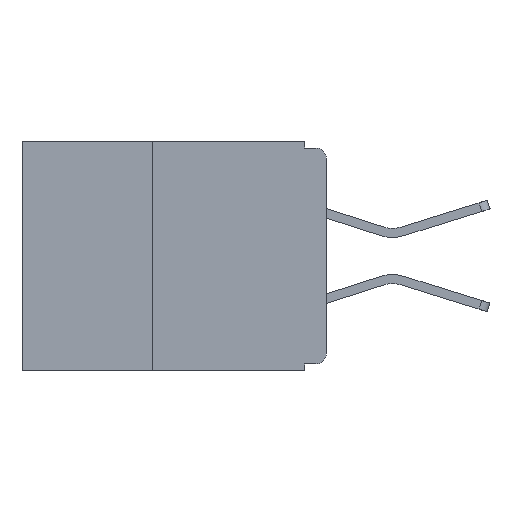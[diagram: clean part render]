
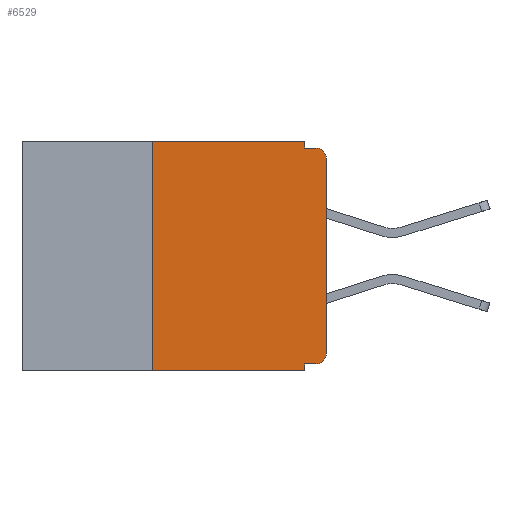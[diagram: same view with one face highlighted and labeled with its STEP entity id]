
A CAD part, left-side view. The second image highlights one B-rep face of the part: STEP entity #6529.
In plain terms, the highlighted planar face has unit normal (-1, 0, 0).
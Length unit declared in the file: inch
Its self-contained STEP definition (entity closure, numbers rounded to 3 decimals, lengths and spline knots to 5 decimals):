
#220 = ORIENTED_EDGE ( 'NONE', *, *, #1841, .T. ) ;
#854 = DIRECTION ( 'NONE',  ( 0., 0., -1. ) ) ;
#867 = CARTESIAN_POINT ( 'NONE',  ( 0., 0.25, -0.33 ) ) ;
#914 = CARTESIAN_POINT ( 'NONE',  ( 0., 0., -0.305 ) ) ;
#943 = DIRECTION ( 'NONE',  ( 0., 0., 1. ) ) ;
#957 = DIRECTION ( 'NONE',  ( -1., 0., 0. ) ) ;
#1030 = CARTESIAN_POINT ( 'NONE',  ( 0., 0.015, -0.305 ) ) ;
#1179 = LINE ( 'NONE', #15894, #25919 ) ;
#1271 = EDGE_CURVE ( 'NONE', #3011, #22748, #14163, .T. ) ;
#1357 = VECTOR ( 'NONE', #10942, 39.37008 ) ;
#1841 = EDGE_CURVE ( 'NONE', #8660, #22748, #8854, .T. ) ;
#1906 = AXIS2_PLACEMENT_3D ( 'NONE', #6302, #23555, #6839 ) ;
#1946 = ORIENTED_EDGE ( 'NONE', *, *, #25654, .T. ) ;
#2000 = CARTESIAN_POINT ( 'NONE',  ( 0., 0.031, 0. ) ) ;
#2890 = VECTOR ( 'NONE', #6925, 39.37008 ) ;
#3011 = VERTEX_POINT ( 'NONE', #15154 ) ;
#3528 = CARTESIAN_POINT ( 'NONE',  ( 0., 0.015, -0.01 ) ) ;
#3566 = EDGE_CURVE ( 'NONE', #28428, #23435, #24831, .T. ) ;
#3914 = DIRECTION ( 'NONE',  ( 0., 0., 1. ) ) ;
#4396 = FACE_OUTER_BOUND ( 'NONE', #19250, .T. ) ;
#4990 = CARTESIAN_POINT ( 'NONE',  ( 0., 0., -0.32 ) ) ;
#5442 = VECTOR ( 'NONE', #26007, 39.37008 ) ;
#5849 = AXIS2_PLACEMENT_3D ( 'NONE', #1030, #957, #854 ) ;
#5925 = ORIENTED_EDGE ( 'NONE', *, *, #29045, .F. ) ;
#6224 = CARTESIAN_POINT ( 'NONE',  ( 0., 0.25, 0. ) ) ;
#6302 = CARTESIAN_POINT ( 'NONE',  ( 0., 0.015, -0.025 ) ) ;
#6384 = EDGE_CURVE ( 'NONE', #9688, #9881, #13815, .T. ) ;
#6529 = ADVANCED_FACE ( 'NONE', ( #4396 ), #29319, .F. ) ;
#6839 = DIRECTION ( 'NONE',  ( 0., 0., -1. ) ) ;
#6925 = DIRECTION ( 'NONE',  ( 0., -1., 0. ) ) ;
#8288 = VECTOR ( 'NONE', #17057, 39.37008 ) ;
#8456 = VECTOR ( 'NONE', #25590, 39.37008 ) ;
#8660 = VERTEX_POINT ( 'NONE', #22276 ) ;
#8854 = CIRCLE ( 'NONE', #1906, 0.015 ) ;
#9190 = LINE ( 'NONE', #13715, #8456 ) ;
#9688 = VERTEX_POINT ( 'NONE', #26473 ) ;
#9698 = DIRECTION ( 'NONE',  ( 0., -1., 0. ) ) ;
#9881 = VERTEX_POINT ( 'NONE', #914 ) ;
#10107 = ORIENTED_EDGE ( 'NONE', *, *, #6384, .T. ) ;
#10459 = ORIENTED_EDGE ( 'NONE', *, *, #1271, .F. ) ;
#10942 = DIRECTION ( 'NONE',  ( 0., -1., 0. ) ) ;
#11364 = VECTOR ( 'NONE', #943, 39.37008 ) ;
#11831 = LINE ( 'NONE', #28255, #5442 ) ;
#12467 = ORIENTED_EDGE ( 'NONE', *, *, #29128, .F. ) ;
#12815 = VERTEX_POINT ( 'NONE', #29385 ) ;
#13604 = ORIENTED_EDGE ( 'NONE', *, *, #22145, .T. ) ;
#13715 = CARTESIAN_POINT ( 'NONE',  ( 0., 0.031, -0.33 ) ) ;
#13815 = CIRCLE ( 'NONE', #5849, 0.015 ) ;
#14163 = LINE ( 'NONE', #21809, #1357 ) ;
#14956 = VERTEX_POINT ( 'NONE', #2000 ) ;
#15154 = CARTESIAN_POINT ( 'NONE',  ( 0., 0.031, -0.01 ) ) ;
#15429 = VECTOR ( 'NONE', #9698, 39.37008 ) ;
#15708 = CARTESIAN_POINT ( 'NONE',  ( 0., 0.031, -0.33 ) ) ;
#15894 = CARTESIAN_POINT ( 'NONE',  ( 0., 0., 0. ) ) ;
#16245 = EDGE_CURVE ( 'NONE', #9688, #12815, #21027, .T. ) ;
#16947 = CARTESIAN_POINT ( 'NONE',  ( 0., 0.437, 0. ) ) ;
#17057 = DIRECTION ( 'NONE',  ( 0., 1., 0. ) ) ;
#17369 = EDGE_CURVE ( 'NONE', #23435, #14956, #25479, .T. ) ;
#17948 = ORIENTED_EDGE ( 'NONE', *, *, #3566, .F. ) ;
#19250 = EDGE_LOOP ( 'NONE', ( #13604, #220, #10459, #12467, #21871, #17948, #1946, #5925, #23321, #10107 ) ) ;
#19499 = VERTEX_POINT ( 'NONE', #15708 ) ;
#20529 = LINE ( 'NONE', #30766, #2890 ) ;
#21027 = LINE ( 'NONE', #4990, #8288 ) ;
#21467 = CARTESIAN_POINT ( 'NONE',  ( 0., 0.25, -0.33 ) ) ;
#21809 = CARTESIAN_POINT ( 'NONE',  ( 0., 0., -0.01 ) ) ;
#21871 = ORIENTED_EDGE ( 'NONE', *, *, #17369, .F. ) ;
#22145 = EDGE_CURVE ( 'NONE', #9881, #8660, #1179, .T. ) ;
#22276 = CARTESIAN_POINT ( 'NONE',  ( 0., 0., -0.025 ) ) ;
#22748 = VERTEX_POINT ( 'NONE', #3528 ) ;
#23321 = ORIENTED_EDGE ( 'NONE', *, *, #16245, .F. ) ;
#23435 = VERTEX_POINT ( 'NONE', #6224 ) ;
#23501 = AXIS2_PLACEMENT_3D ( 'NONE', #29344, #29039, #29016 ) ;
#23555 = DIRECTION ( 'NONE',  ( -1., 0., 0. ) ) ;
#24831 = LINE ( 'NONE', #21467, #11364 ) ;
#25479 = LINE ( 'NONE', #16947, #15429 ) ;
#25590 = DIRECTION ( 'NONE',  ( 0., 0., -1. ) ) ;
#25654 = EDGE_CURVE ( 'NONE', #28428, #19499, #20529, .T. ) ;
#25919 = VECTOR ( 'NONE', #3914, 39.37008 ) ;
#26007 = DIRECTION ( 'NONE',  ( 0., 0., -1. ) ) ;
#26473 = CARTESIAN_POINT ( 'NONE',  ( 0., 0.015, -0.32 ) ) ;
#28255 = CARTESIAN_POINT ( 'NONE',  ( 0., 0.031, 0. ) ) ;
#28428 = VERTEX_POINT ( 'NONE', #867 ) ;
#29016 = DIRECTION ( 'NONE',  ( 0., 0., -1. ) ) ;
#29039 = DIRECTION ( 'NONE',  ( 1., 0., 0. ) ) ;
#29045 = EDGE_CURVE ( 'NONE', #12815, #19499, #9190, .T. ) ;
#29128 = EDGE_CURVE ( 'NONE', #14956, #3011, #11831, .T. ) ;
#29319 = PLANE ( 'NONE',  #23501 ) ;
#29344 = CARTESIAN_POINT ( 'NONE',  ( 0., 0.437, 0. ) ) ;
#29385 = CARTESIAN_POINT ( 'NONE',  ( 0., 0.031, -0.32 ) ) ;
#30766 = CARTESIAN_POINT ( 'NONE',  ( 0., 0.437, -0.33 ) ) ;
